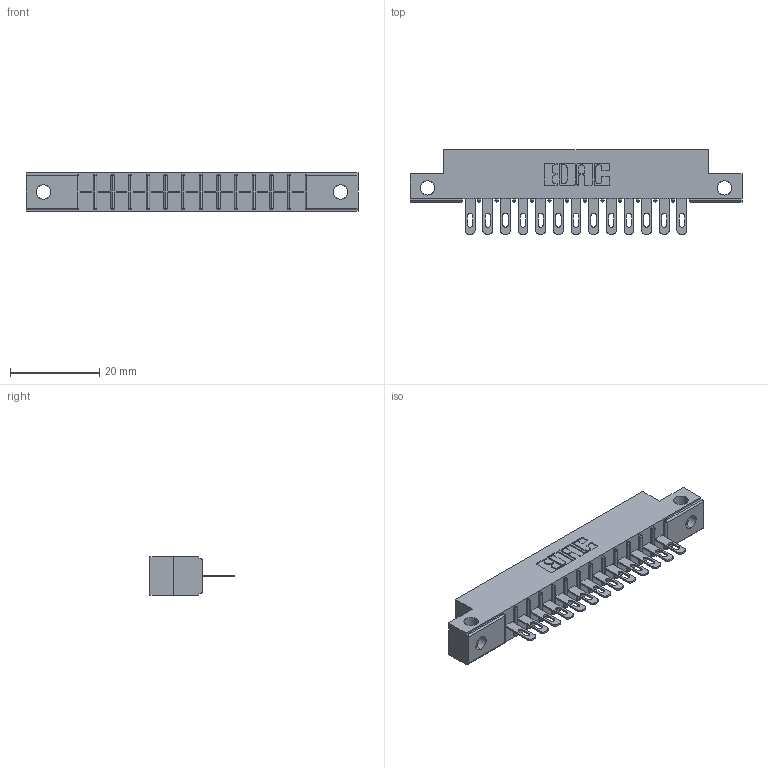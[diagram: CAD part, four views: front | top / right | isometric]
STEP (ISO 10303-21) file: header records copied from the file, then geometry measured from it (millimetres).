
FILE_DESCRIPTION (( 'STEP AP203' ), '1' );
FILE_NAME ('316-013-400-112.STEP', '2020-09-22T16:24:50', ( '' ), ( '' ), 'SwSTEP 2.0', 'SolidWorks 2020', '' );
FILE_SCHEMA (( 'CONFIG_CONTROL_DESIGN' ));
Length unit declared in the file: inch
Products named in the file (3): 316-013-400-112; 306 Part_.128 Dia; 306-290-001_100
Assembly tree (14 placements, depth 2):
  316-013-400-112
    306 Part_.128 Dia
    306-290-001_100  x13
Bounding box: 74.52 x 18.87 x 8.71 mm (x, y, z)
Volume: 4967.4 mm3; surface area: 7203.2 mm2
Topology: 14 solids, 14 shells, 1116 faces, 3147 edges, 2022 vertices
Faces by surface type: plane 718, cylinder 346, sphere 52
Entity records: 16450 total; most frequent: CARTESIAN_POINT 2806, ORIENTED_EDGE 2734, DIRECTION 2709, EDGE_CURVE 1367, VECTOR 1035, LINE 1035, VERTEX_POINT 870, AXIS2_PLACEMENT_3D 837
